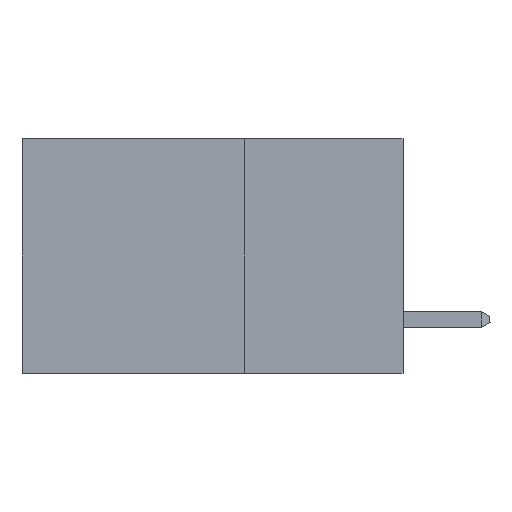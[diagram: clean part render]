
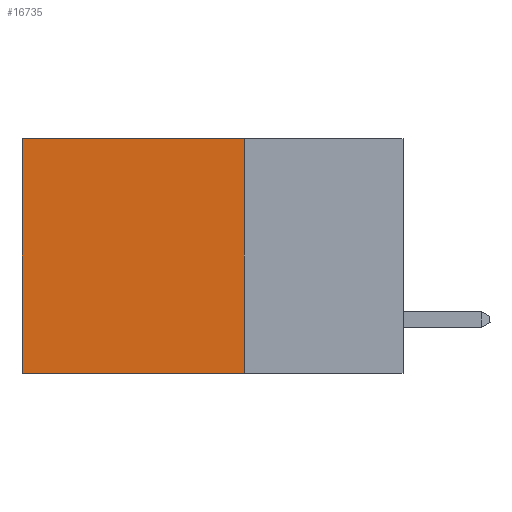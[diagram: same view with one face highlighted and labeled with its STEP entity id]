
A CAD part, left-side view. The second image highlights one B-rep face of the part: STEP entity #16735.
In plain terms, the highlighted planar face has unit normal (-1, 0, 0).
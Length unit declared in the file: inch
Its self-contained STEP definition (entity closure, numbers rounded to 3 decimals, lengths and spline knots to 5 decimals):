
#353 = VERTEX_POINT ( 'NONE', #4159 ) ;
#733 = ORIENTED_EDGE ( 'NONE', *, *, #17857, .T. ) ;
#2318 = LINE ( 'NONE', #27480, #16709 ) ;
#2490 = DIRECTION ( 'NONE',  ( 0., 0., -1. ) ) ;
#3126 = VERTEX_POINT ( 'NONE', #3859 ) ;
#3859 = CARTESIAN_POINT ( 'NONE',  ( 0.2875, 0.25, -0.37 ) ) ;
#4159 = CARTESIAN_POINT ( 'NONE',  ( 0.2875, 0.6, 0. ) ) ;
#4800 = DIRECTION ( 'NONE',  ( 1., 0., 0. ) ) ;
#4837 = CARTESIAN_POINT ( 'NONE',  ( 0.2875, 0.25, 0. ) ) ;
#5649 = VERTEX_POINT ( 'NONE', #14207 ) ;
#7461 = VECTOR ( 'NONE', #25890, 39.37008 ) ;
#14207 = CARTESIAN_POINT ( 'NONE',  ( 0.2875, 0.6, -0.37 ) ) ;
#14220 = ORIENTED_EDGE ( 'NONE', *, *, #21162, .F. ) ;
#14492 = LINE ( 'NONE', #4837, #7461 ) ;
#15165 = FACE_OUTER_BOUND ( 'NONE', #16508, .T. ) ;
#15961 = DIRECTION ( 'NONE',  ( 0., 1., 0. ) ) ;
#16131 = CARTESIAN_POINT ( 'NONE',  ( 0.2875, 0.25, 0. ) ) ;
#16508 = EDGE_LOOP ( 'NONE', ( #733, #26594, #14220, #28448 ) ) ;
#16709 = VECTOR ( 'NONE', #19945, 39.37008 ) ;
#16735 = ADVANCED_FACE ( 'NONE', ( #15165 ), #23118, .F. ) ;
#16938 = VECTOR ( 'NONE', #15961, 39.37008 ) ;
#17857 = EDGE_CURVE ( 'NONE', #353, #5649, #2318, .T. ) ;
#18370 = CARTESIAN_POINT ( 'NONE',  ( 0.2875, 0.25, 0. ) ) ;
#19416 = LINE ( 'NONE', #23659, #16938 ) ;
#19945 = DIRECTION ( 'NONE',  ( 0., 0., -1. ) ) ;
#21162 = EDGE_CURVE ( 'NONE', #24094, #3126, #14492, .T. ) ;
#22228 = VECTOR ( 'NONE', #24538, 39.37008 ) ;
#23118 = PLANE ( 'NONE',  #32689 ) ;
#23659 = CARTESIAN_POINT ( 'NONE',  ( 0.2875, 0.25, -0.37 ) ) ;
#24094 = VERTEX_POINT ( 'NONE', #16131 ) ;
#24538 = DIRECTION ( 'NONE',  ( 0., 1., 0. ) ) ;
#25060 = EDGE_CURVE ( 'NONE', #3126, #5649, #19416, .T. ) ;
#25890 = DIRECTION ( 'NONE',  ( 0., 0., -1. ) ) ;
#26594 = ORIENTED_EDGE ( 'NONE', *, *, #25060, .F. ) ;
#26765 = EDGE_CURVE ( 'NONE', #24094, #353, #27973, .T. ) ;
#27480 = CARTESIAN_POINT ( 'NONE',  ( 0.2875, 0.6, 0. ) ) ;
#27973 = LINE ( 'NONE', #32298, #22228 ) ;
#28448 = ORIENTED_EDGE ( 'NONE', *, *, #26765, .T. ) ;
#32298 = CARTESIAN_POINT ( 'NONE',  ( 0.2875, 0.25, 0. ) ) ;
#32689 = AXIS2_PLACEMENT_3D ( 'NONE', #18370, #4800, #2490 ) ;
